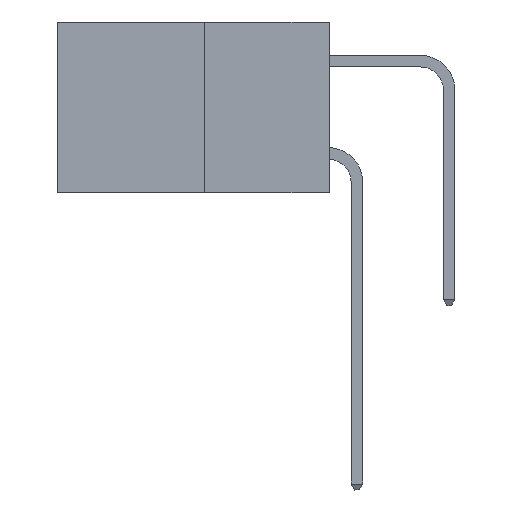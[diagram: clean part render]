
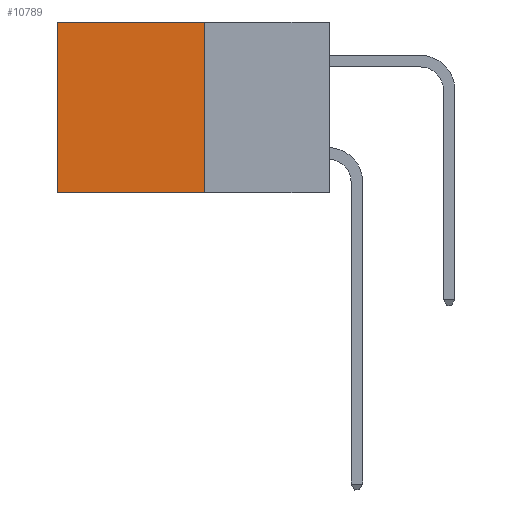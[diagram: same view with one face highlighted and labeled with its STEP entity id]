
A CAD part, left-side view. The second image highlights one B-rep face of the part: STEP entity #10789.
In plain terms, the highlighted planar face has unit normal (-1, 0, 0).
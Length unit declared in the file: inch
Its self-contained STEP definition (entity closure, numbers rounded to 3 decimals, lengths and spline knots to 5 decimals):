
#1041 = ORIENTED_EDGE ( 'NONE', *, *, #18513, .F. ) ;
#1735 = DIRECTION ( 'NONE',  ( 0., 0., -1. ) ) ;
#2341 = CARTESIAN_POINT ( 'NONE',  ( 0.277, 0.27, -0.37 ) ) ;
#2494 = EDGE_CURVE ( 'NONE', #16956, #8637, #4291, .T. ) ;
#2629 = AXIS2_PLACEMENT_3D ( 'NONE', #2341, #12591, #3769 ) ;
#2714 = CARTESIAN_POINT ( 'NONE',  ( 0.277, 0.27, 0. ) ) ;
#3119 = LINE ( 'NONE', #15749, #17563 ) ;
#3578 = ORIENTED_EDGE ( 'NONE', *, *, #14660, .T. ) ;
#3769 = DIRECTION ( 'NONE',  ( 0., 0., -1. ) ) ;
#4291 = LINE ( 'NONE', #8748, #8285 ) ;
#5035 = CARTESIAN_POINT ( 'NONE',  ( 0.277, 0.59, -0.37 ) ) ;
#5281 = CARTESIAN_POINT ( 'NONE',  ( 0.277, 0.59, 0. ) ) ;
#5880 = FACE_OUTER_BOUND ( 'NONE', #11820, .T. ) ;
#5887 = ORIENTED_EDGE ( 'NONE', *, *, #2494, .T. ) ;
#6723 = PLANE ( 'NONE',  #2629 ) ;
#8285 = VECTOR ( 'NONE', #9220, 39.37008 ) ;
#8637 = VERTEX_POINT ( 'NONE', #5281 ) ;
#8748 = CARTESIAN_POINT ( 'NONE',  ( 0.277, 0.27, 0. ) ) ;
#9220 = DIRECTION ( 'NONE',  ( 0., 1., 0. ) ) ;
#9879 = DIRECTION ( 'NONE',  ( 0., 0., -1. ) ) ;
#10252 = EDGE_CURVE ( 'NONE', #16313, #16169, #3119, .T. ) ;
#10552 = CARTESIAN_POINT ( 'NONE',  ( 0.277, 0.27, -0.37 ) ) ;
#10789 = ADVANCED_FACE ( 'NONE', ( #5880 ), #6723, .F. ) ;
#11272 = VECTOR ( 'NONE', #9879, 39.37008 ) ;
#11820 = EDGE_LOOP ( 'NONE', ( #3578, #13954, #1041, #5887 ) ) ;
#12591 = DIRECTION ( 'NONE',  ( 1., 0., 0. ) ) ;
#12921 = DIRECTION ( 'NONE',  ( 0., 1., 0. ) ) ;
#13954 = ORIENTED_EDGE ( 'NONE', *, *, #10252, .F. ) ;
#14132 = CARTESIAN_POINT ( 'NONE',  ( 0.277, 0.27, -0.37 ) ) ;
#14660 = EDGE_CURVE ( 'NONE', #8637, #16169, #15051, .T. ) ;
#14806 = LINE ( 'NONE', #10552, #18429 ) ;
#15051 = LINE ( 'NONE', #15527, #11272 ) ;
#15527 = CARTESIAN_POINT ( 'NONE',  ( 0.277, 0.59, -0.37 ) ) ;
#15749 = CARTESIAN_POINT ( 'NONE',  ( 0.277, 0.27, -0.37 ) ) ;
#16169 = VERTEX_POINT ( 'NONE', #5035 ) ;
#16313 = VERTEX_POINT ( 'NONE', #14132 ) ;
#16956 = VERTEX_POINT ( 'NONE', #2714 ) ;
#17563 = VECTOR ( 'NONE', #12921, 39.37008 ) ;
#18429 = VECTOR ( 'NONE', #1735, 39.37008 ) ;
#18513 = EDGE_CURVE ( 'NONE', #16956, #16313, #14806, .T. ) ;
